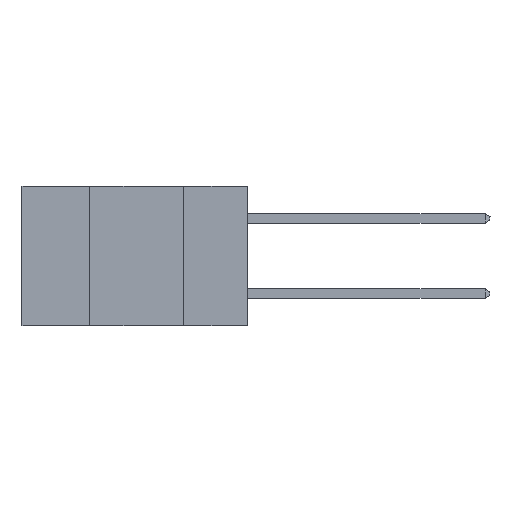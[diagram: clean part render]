
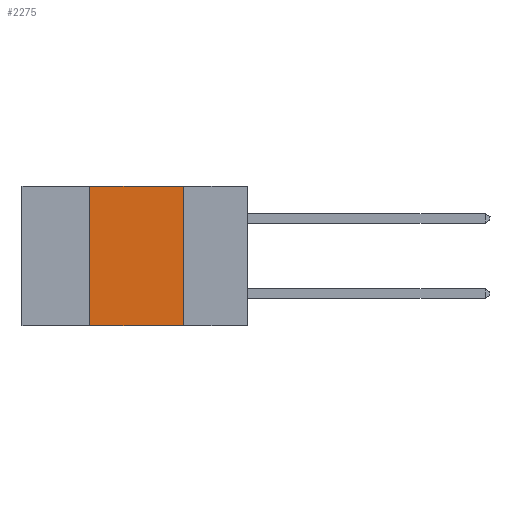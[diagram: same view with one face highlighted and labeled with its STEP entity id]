
A CAD part, left-side view. The second image highlights one B-rep face of the part: STEP entity #2275.
In plain terms, the highlighted planar face has unit normal (-1, 0, 0).
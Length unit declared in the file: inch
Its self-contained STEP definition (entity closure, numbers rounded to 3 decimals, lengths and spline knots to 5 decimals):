
#25 = ORIENTED_EDGE ( 'NONE', *, *, #5537, .F. ) ;
#881 = DIRECTION ( 'NONE',  ( 0., 0., -1. ) ) ;
#934 = CARTESIAN_POINT ( 'NONE',  ( 0., 0.42, -0.37 ) ) ;
#935 = DIRECTION ( 'NONE',  ( 0., 0., -1. ) ) ;
#970 = DIRECTION ( 'NONE',  ( 0., 0., 1. ) ) ;
#2275 = ADVANCED_FACE ( 'NONE', ( #8386 ), #10446, .F. ) ;
#2581 = AXIS2_PLACEMENT_3D ( 'NONE', #2842, #4459, #935 ) ;
#2821 = VERTEX_POINT ( 'NONE', #3128 ) ;
#2842 = CARTESIAN_POINT ( 'NONE',  ( 0., 0.6, 0. ) ) ;
#3029 = VERTEX_POINT ( 'NONE', #12091 ) ;
#3128 = CARTESIAN_POINT ( 'NONE',  ( 0., 0.17, -0.37 ) ) ;
#3598 = LINE ( 'NONE', #10977, #11256 ) ;
#3712 = EDGE_LOOP ( 'NONE', ( #25, #7150, #7203, #10981 ) ) ;
#3930 = EDGE_CURVE ( 'NONE', #4541, #6883, #10541, .T. ) ;
#4174 = CARTESIAN_POINT ( 'NONE',  ( 0., 0.6, -0.37 ) ) ;
#4250 = EDGE_CURVE ( 'NONE', #6883, #3029, #3598, .T. ) ;
#4459 = DIRECTION ( 'NONE',  ( 1., 0., 0. ) ) ;
#4504 = VECTOR ( 'NONE', #881, 39.37008 ) ;
#4541 = VERTEX_POINT ( 'NONE', #934 ) ;
#4641 = VECTOR ( 'NONE', #7166, 39.37008 ) ;
#4672 = CARTESIAN_POINT ( 'NONE',  ( 0., 0.42, -0.37 ) ) ;
#5278 = LINE ( 'NONE', #4174, #4641 ) ;
#5528 = LINE ( 'NONE', #7463, #4504 ) ;
#5537 = EDGE_CURVE ( 'NONE', #3029, #2821, #5528, .T. ) ;
#6883 = VERTEX_POINT ( 'NONE', #11824 ) ;
#7150 = ORIENTED_EDGE ( 'NONE', *, *, #4250, .F. ) ;
#7166 = DIRECTION ( 'NONE',  ( 0., -1., 0. ) ) ;
#7203 = ORIENTED_EDGE ( 'NONE', *, *, #3930, .F. ) ;
#7463 = CARTESIAN_POINT ( 'NONE',  ( 0., 0.17, -0.37 ) ) ;
#8106 = DIRECTION ( 'NONE',  ( 0., -1., 0. ) ) ;
#8386 = FACE_OUTER_BOUND ( 'NONE', #3712, .T. ) ;
#8657 = VECTOR ( 'NONE', #970, 39.37008 ) ;
#10406 = EDGE_CURVE ( 'NONE', #4541, #2821, #5278, .T. ) ;
#10446 = PLANE ( 'NONE',  #2581 ) ;
#10541 = LINE ( 'NONE', #4672, #8657 ) ;
#10977 = CARTESIAN_POINT ( 'NONE',  ( 0., 0.6, 0. ) ) ;
#10981 = ORIENTED_EDGE ( 'NONE', *, *, #10406, .T. ) ;
#11256 = VECTOR ( 'NONE', #8106, 39.37008 ) ;
#11824 = CARTESIAN_POINT ( 'NONE',  ( 0., 0.42, 0. ) ) ;
#12091 = CARTESIAN_POINT ( 'NONE',  ( 0., 0.17, 0. ) ) ;
